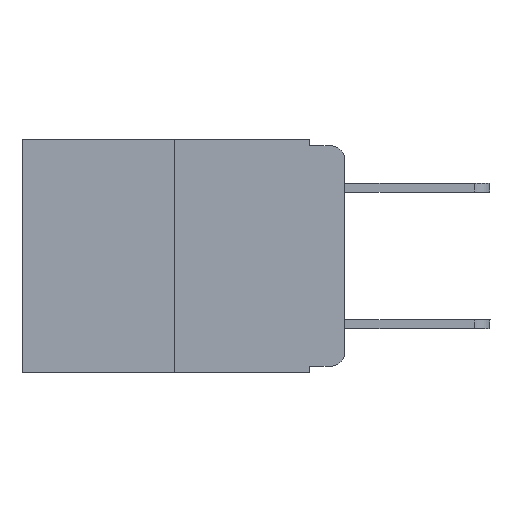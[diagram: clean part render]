
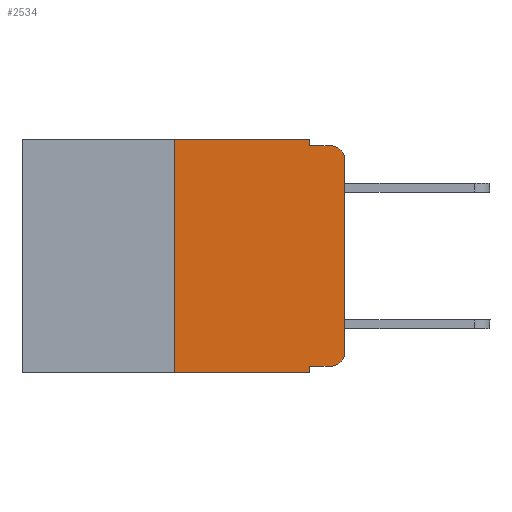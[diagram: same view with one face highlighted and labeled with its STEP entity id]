
A CAD part, left-side view. The second image highlights one B-rep face of the part: STEP entity #2534.
In plain terms, the highlighted planar face has unit normal (-1, 0, 0).
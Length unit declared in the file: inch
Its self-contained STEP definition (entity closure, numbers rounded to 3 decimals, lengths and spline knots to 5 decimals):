
#92 = LINE ( 'NONE', #450, #11382 ) ;
#198 = DIRECTION ( 'NONE',  ( 0., 0., 1. ) ) ;
#243 = ORIENTED_EDGE ( 'NONE', *, *, #14768, .T. ) ;
#400 = CIRCLE ( 'NONE', #1315, 0.02 ) ;
#450 = CARTESIAN_POINT ( 'NONE',  ( 0., 0.051, 0. ) ) ;
#466 = ORIENTED_EDGE ( 'NONE', *, *, #9067, .F. ) ;
#574 = VECTOR ( 'NONE', #12465, 39.37008 ) ;
#1003 = EDGE_CURVE ( 'NONE', #4201, #8542, #92, .T. ) ;
#1066 = CARTESIAN_POINT ( 'NONE',  ( 0., 0.473, 0. ) ) ;
#1078 = CIRCLE ( 'NONE', #4020, 0.02 ) ;
#1166 = ORIENTED_EDGE ( 'NONE', *, *, #8529, .T. ) ;
#1315 = AXIS2_PLACEMENT_3D ( 'NONE', #15001, #14793, #12331 ) ;
#1583 = CARTESIAN_POINT ( 'NONE',  ( 0., 0.02, -0.333 ) ) ;
#1836 = CARTESIAN_POINT ( 'NONE',  ( 0., 0.473, 0. ) ) ;
#2229 = ORIENTED_EDGE ( 'NONE', *, *, #6311, .F. ) ;
#2534 = ADVANCED_FACE ( 'NONE', ( #8468 ), #8378, .F. ) ;
#2653 = VECTOR ( 'NONE', #3771, 39.37008 ) ;
#2793 = CARTESIAN_POINT ( 'NONE',  ( 0., 0.051, -0.333 ) ) ;
#2854 = ORIENTED_EDGE ( 'NONE', *, *, #11601, .T. ) ;
#2909 = DIRECTION ( 'NONE',  ( 0., 0., -1. ) ) ;
#3281 = DIRECTION ( 'NONE',  ( 0., 0., 1. ) ) ;
#3349 = AXIS2_PLACEMENT_3D ( 'NONE', #1066, #10852, #10901 ) ;
#3771 = DIRECTION ( 'NONE',  ( 0., -1., 0. ) ) ;
#3919 = CARTESIAN_POINT ( 'NONE',  ( 0., 0.051, -0.01 ) ) ;
#3959 = CARTESIAN_POINT ( 'NONE',  ( 0., 0.02, -0.01 ) ) ;
#4020 = AXIS2_PLACEMENT_3D ( 'NONE', #15206, #5426, #2909 ) ;
#4172 = CARTESIAN_POINT ( 'NONE',  ( 0., 0., -0.03 ) ) ;
#4201 = VERTEX_POINT ( 'NONE', #5950 ) ;
#4268 = VECTOR ( 'NONE', #3281, 39.37008 ) ;
#5426 = DIRECTION ( 'NONE',  ( -1., 0., 0. ) ) ;
#5587 = CARTESIAN_POINT ( 'NONE',  ( 0., 0.473, -0.343 ) ) ;
#5916 = EDGE_CURVE ( 'NONE', #9347, #12078, #7466, .T. ) ;
#5950 = CARTESIAN_POINT ( 'NONE',  ( 0., 0.051, -0.333 ) ) ;
#6097 = VECTOR ( 'NONE', #9387, 39.37008 ) ;
#6311 = EDGE_CURVE ( 'NONE', #6912, #8373, #10893, .T. ) ;
#6312 = CARTESIAN_POINT ( 'NONE',  ( 0., 0.051, 0. ) ) ;
#6912 = VERTEX_POINT ( 'NONE', #10037 ) ;
#6942 = ORIENTED_EDGE ( 'NONE', *, *, #8435, .T. ) ;
#7466 = LINE ( 'NONE', #1836, #9172 ) ;
#7618 = VECTOR ( 'NONE', #198, 39.37008 ) ;
#7812 = LINE ( 'NONE', #5587, #6097 ) ;
#8373 = VERTEX_POINT ( 'NONE', #3959 ) ;
#8378 = PLANE ( 'NONE',  #3349 ) ;
#8435 = EDGE_CURVE ( 'NONE', #10991, #15284, #1078, .T. ) ;
#8468 = FACE_OUTER_BOUND ( 'NONE', #12257, .T. ) ;
#8529 = EDGE_CURVE ( 'NONE', #15284, #12894, #15836, .T. ) ;
#8542 = VERTEX_POINT ( 'NONE', #11693 ) ;
#8703 = CARTESIAN_POINT ( 'NONE',  ( 0., 0., -0.313 ) ) ;
#8931 = ORIENTED_EDGE ( 'NONE', *, *, #1003, .F. ) ;
#8981 = DIRECTION ( 'NONE',  ( 0., 0., -1. ) ) ;
#9067 = EDGE_CURVE ( 'NONE', #12078, #6912, #13870, .T. ) ;
#9151 = LINE ( 'NONE', #12535, #7618 ) ;
#9172 = VECTOR ( 'NONE', #14148, 39.37008 ) ;
#9347 = VERTEX_POINT ( 'NONE', #9876 ) ;
#9387 = DIRECTION ( 'NONE',  ( 0., -1., 0. ) ) ;
#9876 = CARTESIAN_POINT ( 'NONE',  ( 0., 0.25, 0. ) ) ;
#10037 = CARTESIAN_POINT ( 'NONE',  ( 0., 0.051, -0.01 ) ) ;
#10408 = VECTOR ( 'NONE', #12673, 39.37008 ) ;
#10634 = CARTESIAN_POINT ( 'NONE',  ( 0., 0., 0. ) ) ;
#10792 = ORIENTED_EDGE ( 'NONE', *, *, #15109, .F. ) ;
#10852 = DIRECTION ( 'NONE',  ( 1., 0., 0. ) ) ;
#10886 = EDGE_CURVE ( 'NONE', #12894, #8373, #400, .T. ) ;
#10893 = LINE ( 'NONE', #3919, #2653 ) ;
#10901 = DIRECTION ( 'NONE',  ( 0., 0., -1. ) ) ;
#10991 = VERTEX_POINT ( 'NONE', #1583 ) ;
#11283 = ORIENTED_EDGE ( 'NONE', *, *, #10886, .T. ) ;
#11382 = VECTOR ( 'NONE', #8981, 39.37008 ) ;
#11601 = EDGE_CURVE ( 'NONE', #4201, #10991, #14201, .T. ) ;
#11693 = CARTESIAN_POINT ( 'NONE',  ( 0., 0.051, -0.343 ) ) ;
#12078 = VERTEX_POINT ( 'NONE', #6312 ) ;
#12257 = EDGE_LOOP ( 'NONE', ( #1166, #11283, #2229, #466, #12611, #10792, #243, #8931, #2854, #6942 ) ) ;
#12331 = DIRECTION ( 'NONE',  ( 0., 0., -1. ) ) ;
#12465 = DIRECTION ( 'NONE',  ( 0., -1., 0. ) ) ;
#12535 = CARTESIAN_POINT ( 'NONE',  ( 0., 0.25, 0. ) ) ;
#12611 = ORIENTED_EDGE ( 'NONE', *, *, #5916, .F. ) ;
#12673 = DIRECTION ( 'NONE',  ( 0., 0., -1. ) ) ;
#12827 = CARTESIAN_POINT ( 'NONE',  ( 0., 0.25, -0.343 ) ) ;
#12846 = CARTESIAN_POINT ( 'NONE',  ( 0., 0.051, 0. ) ) ;
#12894 = VERTEX_POINT ( 'NONE', #4172 ) ;
#13870 = LINE ( 'NONE', #12846, #10408 ) ;
#14148 = DIRECTION ( 'NONE',  ( 0., -1., 0. ) ) ;
#14201 = LINE ( 'NONE', #2793, #574 ) ;
#14768 = EDGE_CURVE ( 'NONE', #15743, #8542, #7812, .T. ) ;
#14793 = DIRECTION ( 'NONE',  ( -1., 0., 0. ) ) ;
#15001 = CARTESIAN_POINT ( 'NONE',  ( 0., 0.02, -0.03 ) ) ;
#15109 = EDGE_CURVE ( 'NONE', #15743, #9347, #9151, .T. ) ;
#15206 = CARTESIAN_POINT ( 'NONE',  ( 0., 0.02, -0.313 ) ) ;
#15284 = VERTEX_POINT ( 'NONE', #8703 ) ;
#15743 = VERTEX_POINT ( 'NONE', #12827 ) ;
#15836 = LINE ( 'NONE', #10634, #4268 ) ;
